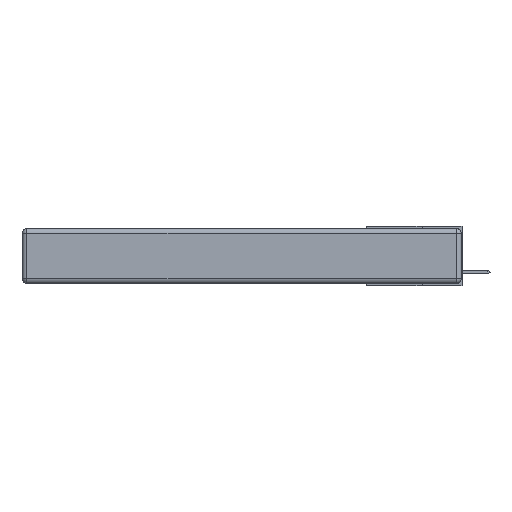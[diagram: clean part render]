
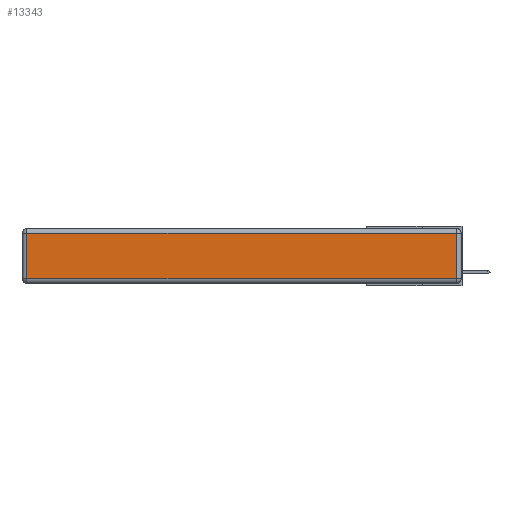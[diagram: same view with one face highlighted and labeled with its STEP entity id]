
A CAD part, left-side view. The second image highlights one B-rep face of the part: STEP entity #13343.
In plain terms, the highlighted planar face has unit normal (-1, 0, 0).
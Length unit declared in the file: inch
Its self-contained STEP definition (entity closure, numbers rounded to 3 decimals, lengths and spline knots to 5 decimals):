
#145 = VECTOR ( 'NONE', #15424, 39.37008 ) ;
#1256 = CARTESIAN_POINT ( 'NONE',  ( 0., 2.72, -0.313 ) ) ;
#2204 = DIRECTION ( 'NONE',  ( 0., 0., 1. ) ) ;
#2305 = DIRECTION ( 'NONE',  ( 0., 0., -1. ) ) ;
#3549 = EDGE_CURVE ( 'NONE', #10757, #19152, #11169, .T. ) ;
#3902 = VECTOR ( 'NONE', #18183, 39.37008 ) ;
#4611 = PLANE ( 'NONE',  #19340 ) ;
#4714 = DIRECTION ( 'NONE',  ( -1., 0., 0. ) ) ;
#5075 = CARTESIAN_POINT ( 'NONE',  ( 0., 2.75, -0.03 ) ) ;
#8362 = ORIENTED_EDGE ( 'NONE', *, *, #16245, .T. ) ;
#9539 = DIRECTION ( 'NONE',  ( 0., 1., 0. ) ) ;
#9544 = EDGE_CURVE ( 'NONE', #20617, #10757, #11529, .T. ) ;
#10757 = VERTEX_POINT ( 'NONE', #24398 ) ;
#10839 = VERTEX_POINT ( 'NONE', #1256 ) ;
#10841 = VECTOR ( 'NONE', #9539, 39.37008 ) ;
#11169 = LINE ( 'NONE', #5075, #10841 ) ;
#11386 = EDGE_LOOP ( 'NONE', ( #8362, #14412, #19417, #20983 ) ) ;
#11387 = CARTESIAN_POINT ( 'NONE',  ( 0., 2.72, -0.343 ) ) ;
#11529 = LINE ( 'NONE', #11848, #3902 ) ;
#11848 = CARTESIAN_POINT ( 'NONE',  ( 0., 0.03, -0.343 ) ) ;
#13340 = EDGE_CURVE ( 'NONE', #19152, #10839, #19903, .T. ) ;
#13343 = ADVANCED_FACE ( 'NONE', ( #28148 ), #4611, .T. ) ;
#14412 = ORIENTED_EDGE ( 'NONE', *, *, #9544, .T. ) ;
#15424 = DIRECTION ( 'NONE',  ( 0., -1., 0. ) ) ;
#16245 = EDGE_CURVE ( 'NONE', #10839, #20617, #19819, .T. ) ;
#18183 = DIRECTION ( 'NONE',  ( 0., 0., 1. ) ) ;
#18899 = CARTESIAN_POINT ( 'NONE',  ( 0., 2.72, -0.03 ) ) ;
#19152 = VERTEX_POINT ( 'NONE', #18899 ) ;
#19340 = AXIS2_PLACEMENT_3D ( 'NONE', #24637, #4714, #2204 ) ;
#19417 = ORIENTED_EDGE ( 'NONE', *, *, #3549, .T. ) ;
#19819 = LINE ( 'NONE', #28466, #145 ) ;
#19903 = LINE ( 'NONE', #11387, #27820 ) ;
#20617 = VERTEX_POINT ( 'NONE', #20834 ) ;
#20834 = CARTESIAN_POINT ( 'NONE',  ( 0., 0.03, -0.313 ) ) ;
#20983 = ORIENTED_EDGE ( 'NONE', *, *, #13340, .T. ) ;
#24398 = CARTESIAN_POINT ( 'NONE',  ( 0., 0.03, -0.03 ) ) ;
#24637 = CARTESIAN_POINT ( 'NONE',  ( 0., 0., -0.343 ) ) ;
#27820 = VECTOR ( 'NONE', #2305, 39.37008 ) ;
#28148 = FACE_OUTER_BOUND ( 'NONE', #11386, .T. ) ;
#28466 = CARTESIAN_POINT ( 'NONE',  ( 0., 0., -0.313 ) ) ;
